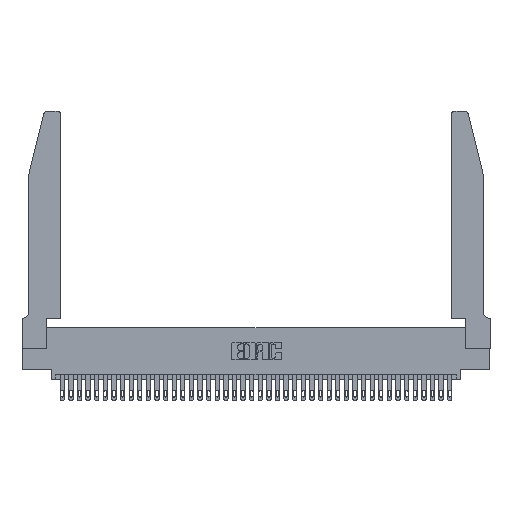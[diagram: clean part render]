
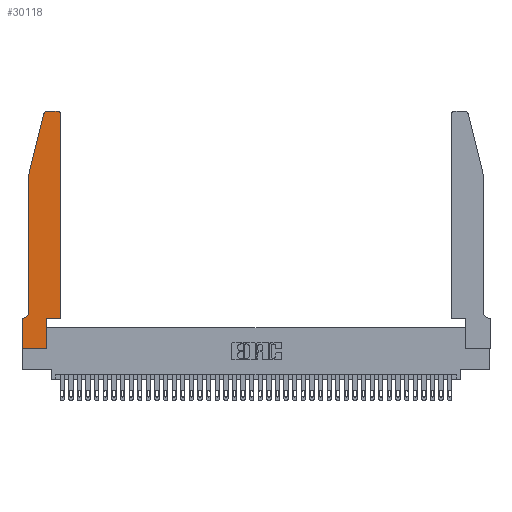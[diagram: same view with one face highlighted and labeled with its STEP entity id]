
A CAD part, top view. The second image highlights one B-rep face of the part: STEP entity #30118.
In plain terms, the highlighted planar face has unit normal (0, 0, 1).
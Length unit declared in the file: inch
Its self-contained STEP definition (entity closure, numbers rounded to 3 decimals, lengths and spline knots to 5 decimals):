
#268 = VERTEX_POINT ( 'NONE', #31288 ) ;
#755 = LINE ( 'NONE', #23990, #40356 ) ;
#1034 = LINE ( 'NONE', #38442, #23547 ) ;
#1084 = DIRECTION ( 'NONE',  ( 0., -1., 0. ) ) ;
#1108 = CIRCLE ( 'NONE', #19508, 0.07 ) ;
#1680 = ORIENTED_EDGE ( 'NONE', *, *, #29099, .T. ) ;
#2976 = CARTESIAN_POINT ( 'NONE',  ( 0.4205, 2.72, 0.37 ) ) ;
#3182 = DIRECTION ( 'NONE',  ( -0.239, -0.971, 0. ) ) ;
#3775 = EDGE_CURVE ( 'NONE', #34730, #22027, #19129, .T. ) ;
#3904 = CARTESIAN_POINT ( 'NONE',  ( 0.4205, 2.75, 0.37 ) ) ;
#3936 = CARTESIAN_POINT ( 'NONE',  ( 0.25487, 2.72718, 0.37 ) ) ;
#4078 = ORIENTED_EDGE ( 'NONE', *, *, #25411, .T. ) ;
#4318 = ORIENTED_EDGE ( 'NONE', *, *, #12941, .T. ) ;
#5668 = DIRECTION ( 'NONE',  ( 0., 0., 1. ) ) ;
#5774 = DIRECTION ( 'NONE',  ( -1., 0., 0. ) ) ;
#6191 = DIRECTION ( 'NONE',  ( 1., 0., 0. ) ) ;
#7153 = ORIENTED_EDGE ( 'NONE', *, *, #28956, .T. ) ;
#7409 = VECTOR ( 'NONE', #3182, 39.37008 ) ;
#7431 = EDGE_CURVE ( 'NONE', #16099, #33611, #15635, .T. ) ;
#7574 = CARTESIAN_POINT ( 'NONE',  ( 0., 0.35, 0.37 ) ) ;
#9016 = DIRECTION ( 'NONE',  ( 0., 0., 1. ) ) ;
#9733 = CARTESIAN_POINT ( 'NONE',  ( 0.4505, 0.35, 0.37 ) ) ;
#10428 = EDGE_CURVE ( 'NONE', #11412, #32197, #755, .T. ) ;
#10868 = VECTOR ( 'NONE', #26384, 39.37008 ) ;
#11136 = LINE ( 'NONE', #25702, #37435 ) ;
#11191 = EDGE_CURVE ( 'NONE', #33611, #21231, #25550, .T. ) ;
#11412 = VERTEX_POINT ( 'NONE', #22752 ) ;
#12287 = DIRECTION ( 'NONE',  ( 1., 0., 0. ) ) ;
#12646 = ORIENTED_EDGE ( 'NONE', *, *, #33656, .T. ) ;
#12941 = EDGE_CURVE ( 'NONE', #23555, #18553, #26106, .T. ) ;
#13154 = CARTESIAN_POINT ( 'NONE',  ( 0.2865, 0., 0.37 ) ) ;
#13570 = DIRECTION ( 'NONE',  ( -1., 0., 0. ) ) ;
#14472 = ORIENTED_EDGE ( 'NONE', *, *, #28268, .T. ) ;
#14546 = LINE ( 'NONE', #21544, #21829 ) ;
#14765 = ORIENTED_EDGE ( 'NONE', *, *, #10428, .T. ) ;
#14822 = CARTESIAN_POINT ( 'NONE',  ( 0., 0.35, 0.37 ) ) ;
#15337 = CARTESIAN_POINT ( 'NONE',  ( 0.0055, 0.42, 0.37 ) ) ;
#15635 = LINE ( 'NONE', #31441, #19009 ) ;
#16006 = ORIENTED_EDGE ( 'NONE', *, *, #11191, .T. ) ;
#16099 = VERTEX_POINT ( 'NONE', #3904 ) ;
#16173 = CARTESIAN_POINT ( 'NONE',  ( 0., 0., 0.37 ) ) ;
#16458 = DIRECTION ( 'NONE',  ( 0., 1., 0. ) ) ;
#17002 = EDGE_CURVE ( 'NONE', #22027, #37779, #11136, .T. ) ;
#17710 = ORIENTED_EDGE ( 'NONE', *, *, #17002, .T. ) ;
#17794 = DIRECTION ( 'NONE',  ( 0., 0., 1. ) ) ;
#17854 = VECTOR ( 'NONE', #13570, 39.37008 ) ;
#18279 = CARTESIAN_POINT ( 'NONE',  ( 0.0055, 0.35, 0.37 ) ) ;
#18454 = CARTESIAN_POINT ( 'NONE',  ( 0.284, 2.75, 0.37 ) ) ;
#18553 = VERTEX_POINT ( 'NONE', #7574 ) ;
#19009 = VECTOR ( 'NONE', #34531, 39.37008 ) ;
#19129 = LINE ( 'NONE', #16173, #10868 ) ;
#19508 = AXIS2_PLACEMENT_3D ( 'NONE', #15337, #27445, #5774 ) ;
#20452 = CARTESIAN_POINT ( 'NONE',  ( 0.0755, 0.42, 0.37 ) ) ;
#20664 = ORIENTED_EDGE ( 'NONE', *, *, #33270, .T. ) ;
#21231 = VERTEX_POINT ( 'NONE', #3936 ) ;
#21544 = CARTESIAN_POINT ( 'NONE',  ( 0.4505, 0.35, 0.37 ) ) ;
#21829 = VECTOR ( 'NONE', #34044, 39.37008 ) ;
#22027 = VERTEX_POINT ( 'NONE', #13154 ) ;
#22752 = CARTESIAN_POINT ( 'NONE',  ( 0.0755, 2., 0.37 ) ) ;
#23547 = VECTOR ( 'NONE', #1084, 39.37008 ) ;
#23555 = VERTEX_POINT ( 'NONE', #18279 ) ;
#23990 = CARTESIAN_POINT ( 'NONE',  ( 0.0755, 2., 0.37 ) ) ;
#24673 = AXIS2_PLACEMENT_3D ( 'NONE', #2976, #9016, #12287 ) ;
#24856 = CARTESIAN_POINT ( 'NONE',  ( 0.284, 2.72, 0.37 ) ) ;
#25411 = EDGE_CURVE ( 'NONE', #37779, #268, #14546, .T. ) ;
#25550 = CIRCLE ( 'NONE', #28132, 0.03 ) ;
#25702 = CARTESIAN_POINT ( 'NONE',  ( 0.2865, 0.35, 0.37 ) ) ;
#25738 = ORIENTED_EDGE ( 'NONE', *, *, #3775, .T. ) ;
#26106 = LINE ( 'NONE', #26323, #17854 ) ;
#26323 = CARTESIAN_POINT ( 'NONE',  ( 0.0755, 0.35, 0.37 ) ) ;
#26384 = DIRECTION ( 'NONE',  ( 1., 0., 0. ) ) ;
#27047 = PLANE ( 'NONE',  #27822 ) ;
#27255 = DIRECTION ( 'NONE',  ( 0., -1., 0. ) ) ;
#27325 = DIRECTION ( 'NONE',  ( 1., 0., 0. ) ) ;
#27445 = DIRECTION ( 'NONE',  ( 0., 0., -1. ) ) ;
#27822 = AXIS2_PLACEMENT_3D ( 'NONE', #14822, #17794, #27325 ) ;
#27911 = ORIENTED_EDGE ( 'NONE', *, *, #7431, .T. ) ;
#28132 = AXIS2_PLACEMENT_3D ( 'NONE', #24856, #5668, #6191 ) ;
#28268 = EDGE_CURVE ( 'NONE', #21231, #11412, #28850, .T. ) ;
#28849 = CIRCLE ( 'NONE', #24673, 0.03 ) ;
#28850 = LINE ( 'NONE', #34366, #7409 ) ;
#28946 = LINE ( 'NONE', #9733, #36298 ) ;
#28956 = EDGE_CURVE ( 'NONE', #18553, #34730, #1034, .T. ) ;
#29099 = EDGE_CURVE ( 'NONE', #36142, #16099, #28849, .T. ) ;
#30118 = ADVANCED_FACE ( 'NONE', ( #32742 ), #27047, .T. ) ;
#31288 = CARTESIAN_POINT ( 'NONE',  ( 0.4505, 0.35, 0.37 ) ) ;
#31441 = CARTESIAN_POINT ( 'NONE',  ( 0.2605, 2.75, 0.37 ) ) ;
#32197 = VERTEX_POINT ( 'NONE', #20452 ) ;
#32742 = FACE_OUTER_BOUND ( 'NONE', #39186, .T. ) ;
#32867 = CARTESIAN_POINT ( 'NONE',  ( 0., 0., 0.37 ) ) ;
#33270 = EDGE_CURVE ( 'NONE', #268, #36142, #28946, .T. ) ;
#33611 = VERTEX_POINT ( 'NONE', #18454 ) ;
#33656 = EDGE_CURVE ( 'NONE', #32197, #23555, #1108, .T. ) ;
#34044 = DIRECTION ( 'NONE',  ( 1., 0., 0. ) ) ;
#34366 = CARTESIAN_POINT ( 'NONE',  ( 0.0755, 2., 0.37 ) ) ;
#34531 = DIRECTION ( 'NONE',  ( -1., 0., 0. ) ) ;
#34615 = DIRECTION ( 'NONE',  ( 0., 1., 0. ) ) ;
#34730 = VERTEX_POINT ( 'NONE', #32867 ) ;
#36142 = VERTEX_POINT ( 'NONE', #36603 ) ;
#36298 = VECTOR ( 'NONE', #34615, 39.37008 ) ;
#36603 = CARTESIAN_POINT ( 'NONE',  ( 0.4505, 2.72, 0.37 ) ) ;
#37435 = VECTOR ( 'NONE', #16458, 39.37008 ) ;
#37779 = VERTEX_POINT ( 'NONE', #39086 ) ;
#38442 = CARTESIAN_POINT ( 'NONE',  ( 0., 0., 0.37 ) ) ;
#39086 = CARTESIAN_POINT ( 'NONE',  ( 0.2865, 0.35, 0.37 ) ) ;
#39186 = EDGE_LOOP ( 'NONE', ( #27911, #16006, #14472, #14765, #12646, #4318, #7153, #25738, #17710, #4078, #20664, #1680 ) ) ;
#40356 = VECTOR ( 'NONE', #27255, 39.37008 ) ;
